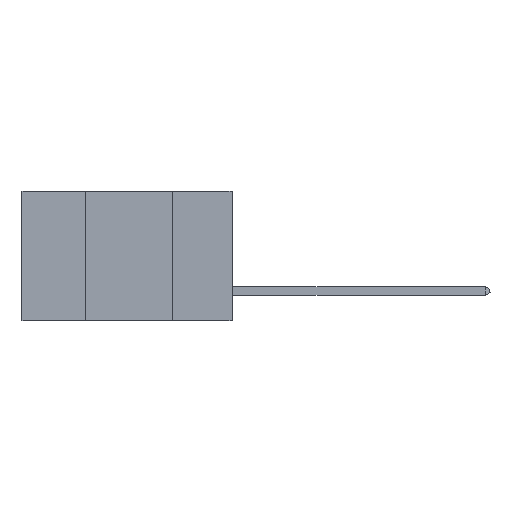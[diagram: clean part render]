
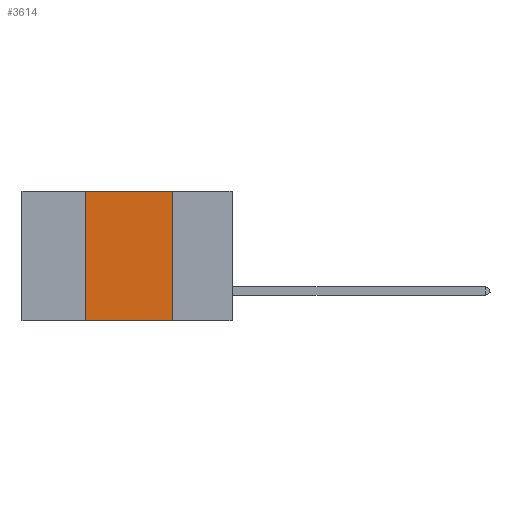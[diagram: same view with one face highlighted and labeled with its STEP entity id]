
A CAD part, left-side view. The second image highlights one B-rep face of the part: STEP entity #3614.
In plain terms, the highlighted planar face has unit normal (-1, 0, 0).
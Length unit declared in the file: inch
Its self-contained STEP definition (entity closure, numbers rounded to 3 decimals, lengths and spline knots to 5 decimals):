
#1 = CARTESIAN_POINT ( 'NONE',  ( 0., 0.6, 0. ) ) ;
#355 = LINE ( 'NONE', #8967, #5749 ) ;
#400 = EDGE_CURVE ( 'NONE', #999, #3041, #3611, .T. ) ;
#839 = DIRECTION ( 'NONE',  ( 1., 0., 0. ) ) ;
#999 = VERTEX_POINT ( 'NONE', #9390 ) ;
#1854 = LINE ( 'NONE', #1, #7501 ) ;
#1954 = VERTEX_POINT ( 'NONE', #9297 ) ;
#2002 = VECTOR ( 'NONE', #7422, 39.37008 ) ;
#2130 = LINE ( 'NONE', #5838, #2002 ) ;
#2189 = ORIENTED_EDGE ( 'NONE', *, *, #400, .F. ) ;
#2580 = EDGE_CURVE ( 'NONE', #5497, #999, #1854, .T. ) ;
#2583 = DIRECTION ( 'NONE',  ( 0., -1., 0. ) ) ;
#3041 = VERTEX_POINT ( 'NONE', #9106 ) ;
#3611 = LINE ( 'NONE', #9716, #8881 ) ;
#3614 = ADVANCED_FACE ( 'NONE', ( #5298 ), #5275, .F. ) ;
#4198 = EDGE_LOOP ( 'NONE', ( #2189, #4361, #8950, #6250 ) ) ;
#4361 = ORIENTED_EDGE ( 'NONE', *, *, #2580, .F. ) ;
#5275 = PLANE ( 'NONE',  #8464 ) ;
#5298 = FACE_OUTER_BOUND ( 'NONE', #4198, .T. ) ;
#5497 = VERTEX_POINT ( 'NONE', #8671 ) ;
#5646 = EDGE_CURVE ( 'NONE', #1954, #3041, #355, .T. ) ;
#5749 = VECTOR ( 'NONE', #2583, 39.37008 ) ;
#5838 = CARTESIAN_POINT ( 'NONE',  ( 0., 0.42, 0. ) ) ;
#6159 = CARTESIAN_POINT ( 'NONE',  ( 0., 0.6, 0. ) ) ;
#6210 = DIRECTION ( 'NONE',  ( 0., -1., 0. ) ) ;
#6250 = ORIENTED_EDGE ( 'NONE', *, *, #5646, .T. ) ;
#6329 = DIRECTION ( 'NONE',  ( 0., 0., -1. ) ) ;
#6645 = DIRECTION ( 'NONE',  ( 0., 0., -1. ) ) ;
#7422 = DIRECTION ( 'NONE',  ( 0., 0., 1. ) ) ;
#7501 = VECTOR ( 'NONE', #6210, 39.37008 ) ;
#7803 = EDGE_CURVE ( 'NONE', #1954, #5497, #2130, .T. ) ;
#8464 = AXIS2_PLACEMENT_3D ( 'NONE', #6159, #839, #6329 ) ;
#8671 = CARTESIAN_POINT ( 'NONE',  ( 0., 0.42, 0. ) ) ;
#8881 = VECTOR ( 'NONE', #6645, 39.37008 ) ;
#8950 = ORIENTED_EDGE ( 'NONE', *, *, #7803, .F. ) ;
#8967 = CARTESIAN_POINT ( 'NONE',  ( 0., 0.6, -0.37 ) ) ;
#9106 = CARTESIAN_POINT ( 'NONE',  ( 0., 0.17, -0.37 ) ) ;
#9297 = CARTESIAN_POINT ( 'NONE',  ( 0., 0.42, -0.37 ) ) ;
#9390 = CARTESIAN_POINT ( 'NONE',  ( 0., 0.17, 0. ) ) ;
#9716 = CARTESIAN_POINT ( 'NONE',  ( 0., 0.17, 0. ) ) ;
